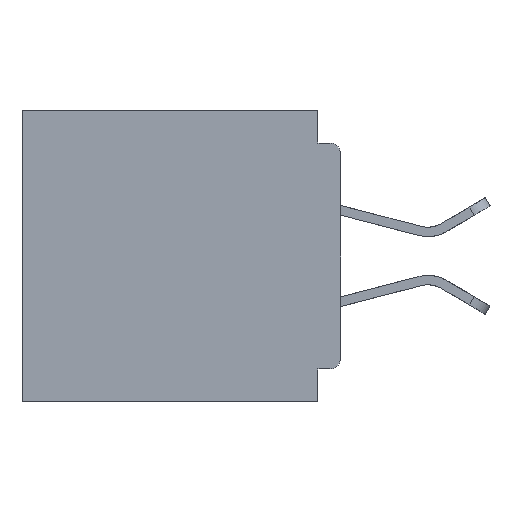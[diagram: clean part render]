
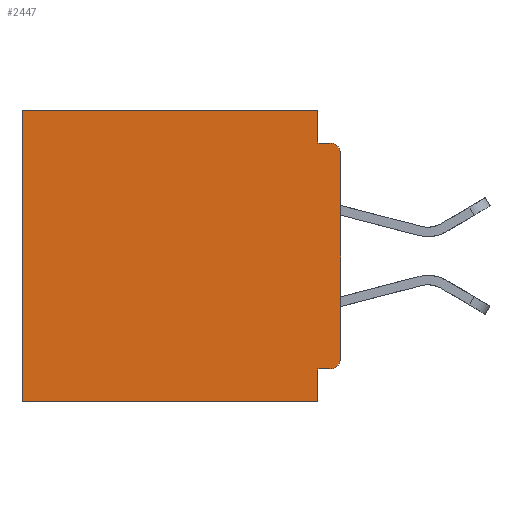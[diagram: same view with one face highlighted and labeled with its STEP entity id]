
A CAD part, left-side view. The second image highlights one B-rep face of the part: STEP entity #2447.
In plain terms, the highlighted planar face has unit normal (-1, 0, 0).
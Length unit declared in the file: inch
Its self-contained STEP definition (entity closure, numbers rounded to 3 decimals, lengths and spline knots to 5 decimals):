
#184 = CARTESIAN_POINT ( 'NONE',  ( 0.3, 0.015, -0.06 ) ) ;
#688 = CARTESIAN_POINT ( 'NONE',  ( 0.3, 0.437, -0.4 ) ) ;
#693 = LINE ( 'NONE', #8231, #17201 ) ;
#1310 = VERTEX_POINT ( 'NONE', #15834 ) ;
#2065 = CARTESIAN_POINT ( 'NONE',  ( 0.3, 0.031, 0. ) ) ;
#2311 = ORIENTED_EDGE ( 'NONE', *, *, #19249, .T. ) ;
#2447 = ADVANCED_FACE ( 'NONE', ( #35693 ), #14220, .F. ) ;
#3426 = CARTESIAN_POINT ( 'NONE',  ( 0.3, 0.437, 0. ) ) ;
#3499 = DIRECTION ( 'NONE',  ( 0., 0., -1. ) ) ;
#3532 = LINE ( 'NONE', #29612, #12281 ) ;
#3850 = ORIENTED_EDGE ( 'NONE', *, *, #18286, .T. ) ;
#3914 = VECTOR ( 'NONE', #31514, 39.37008 ) ;
#6307 = VECTOR ( 'NONE', #27047, 39.37008 ) ;
#6493 = EDGE_CURVE ( 'NONE', #14926, #7414, #3532, .T. ) ;
#6850 = CIRCLE ( 'NONE', #20742, 0.015 ) ;
#7414 = VERTEX_POINT ( 'NONE', #33051 ) ;
#7679 = VERTEX_POINT ( 'NONE', #27681 ) ;
#7861 = ORIENTED_EDGE ( 'NONE', *, *, #28051, .F. ) ;
#8055 = LINE ( 'NONE', #41346, #25611 ) ;
#8152 = VERTEX_POINT ( 'NONE', #17889 ) ;
#8231 = CARTESIAN_POINT ( 'NONE',  ( 0.3, 0., 0. ) ) ;
#8376 = CARTESIAN_POINT ( 'NONE',  ( 0.3, 0.031, 0. ) ) ;
#8762 = CARTESIAN_POINT ( 'NONE',  ( 0.3, 0., -0.4 ) ) ;
#9090 = LINE ( 'NONE', #11339, #25599 ) ;
#9345 = CARTESIAN_POINT ( 'NONE',  ( 0.3, 0., -0.4 ) ) ;
#10101 = DIRECTION ( 'NONE',  ( 1., 0., 0. ) ) ;
#10791 = AXIS2_PLACEMENT_3D ( 'NONE', #184, #23217, #3499 ) ;
#11339 = CARTESIAN_POINT ( 'NONE',  ( 0.3, 0., -0.355 ) ) ;
#11395 = EDGE_CURVE ( 'NONE', #7679, #1310, #9090, .T. ) ;
#11830 = CARTESIAN_POINT ( 'NONE',  ( 0.3, 0., -0.4 ) ) ;
#12067 = DIRECTION ( 'NONE',  ( 0., 0., -1. ) ) ;
#12228 = DIRECTION ( 'NONE',  ( -1., 0., 0. ) ) ;
#12281 = VECTOR ( 'NONE', #29844, 39.37008 ) ;
#12708 = ORIENTED_EDGE ( 'NONE', *, *, #35190, .F. ) ;
#12833 = ORIENTED_EDGE ( 'NONE', *, *, #25616, .F. ) ;
#13420 = VERTEX_POINT ( 'NONE', #3426 ) ;
#14220 = PLANE ( 'NONE',  #16110 ) ;
#14256 = ORIENTED_EDGE ( 'NONE', *, *, #11395, .F. ) ;
#14680 = DIRECTION ( 'NONE',  ( 0., 1., 0. ) ) ;
#14926 = VERTEX_POINT ( 'NONE', #34798 ) ;
#15834 = CARTESIAN_POINT ( 'NONE',  ( 0.3, 0.031, -0.355 ) ) ;
#16017 = DIRECTION ( 'NONE',  ( 0., 0., -1. ) ) ;
#16110 = AXIS2_PLACEMENT_3D ( 'NONE', #8762, #10101, #16213 ) ;
#16213 = DIRECTION ( 'NONE',  ( 0., 0., -1. ) ) ;
#16778 = VERTEX_POINT ( 'NONE', #8376 ) ;
#17102 = EDGE_CURVE ( 'NONE', #36578, #7414, #20330, .T. ) ;
#17201 = VECTOR ( 'NONE', #24676, 39.37008 ) ;
#17889 = CARTESIAN_POINT ( 'NONE',  ( 0.3, 0.031, -0.4 ) ) ;
#18135 = VECTOR ( 'NONE', #16017, 39.37008 ) ;
#18279 = VERTEX_POINT ( 'NONE', #31077 ) ;
#18286 = EDGE_CURVE ( 'NONE', #16778, #13420, #693, .T. ) ;
#18550 = CARTESIAN_POINT ( 'NONE',  ( 0.3, 0.437, -0.4 ) ) ;
#19187 = LINE ( 'NONE', #9345, #18135 ) ;
#19249 = EDGE_CURVE ( 'NONE', #13420, #19551, #41092, .T. ) ;
#19551 = VERTEX_POINT ( 'NONE', #18550 ) ;
#20330 = CIRCLE ( 'NONE', #10791, 0.015 ) ;
#20397 = LINE ( 'NONE', #2065, #3914 ) ;
#20742 = AXIS2_PLACEMENT_3D ( 'NONE', #31883, #12228, #35134 ) ;
#23217 = DIRECTION ( 'NONE',  ( -1., 0., 0. ) ) ;
#23255 = VECTOR ( 'NONE', #31499, 39.37008 ) ;
#24676 = DIRECTION ( 'NONE',  ( 0., 1., 0. ) ) ;
#25599 = VECTOR ( 'NONE', #14680, 39.37008 ) ;
#25611 = VECTOR ( 'NONE', #12067, 39.37008 ) ;
#25616 = EDGE_CURVE ( 'NONE', #36578, #18279, #19187, .T. ) ;
#26516 = CARTESIAN_POINT ( 'NONE',  ( 0.3, 0., -0.06 ) ) ;
#27047 = DIRECTION ( 'NONE',  ( 0., 0., -1. ) ) ;
#27308 = ORIENTED_EDGE ( 'NONE', *, *, #6493, .F. ) ;
#27681 = CARTESIAN_POINT ( 'NONE',  ( 0.3, 0.015, -0.355 ) ) ;
#28051 = EDGE_CURVE ( 'NONE', #16778, #14926, #20397, .T. ) ;
#28535 = EDGE_LOOP ( 'NONE', ( #12833, #32871, #27308, #7861, #3850, #2311, #35212, #12708, #14256, #42350 ) ) ;
#29612 = CARTESIAN_POINT ( 'NONE',  ( 0.3, 0., -0.045 ) ) ;
#29844 = DIRECTION ( 'NONE',  ( 0., -1., 0. ) ) ;
#31077 = CARTESIAN_POINT ( 'NONE',  ( 0.3, 0., -0.34 ) ) ;
#31260 = EDGE_CURVE ( 'NONE', #8152, #19551, #31941, .T. ) ;
#31499 = DIRECTION ( 'NONE',  ( 0., 1., 0. ) ) ;
#31514 = DIRECTION ( 'NONE',  ( 0., 0., -1. ) ) ;
#31883 = CARTESIAN_POINT ( 'NONE',  ( 0.3, 0.015, -0.34 ) ) ;
#31941 = LINE ( 'NONE', #11830, #23255 ) ;
#32871 = ORIENTED_EDGE ( 'NONE', *, *, #17102, .T. ) ;
#33051 = CARTESIAN_POINT ( 'NONE',  ( 0.3, 0.015, -0.045 ) ) ;
#34798 = CARTESIAN_POINT ( 'NONE',  ( 0.3, 0.031, -0.045 ) ) ;
#35134 = DIRECTION ( 'NONE',  ( 0., 0., -1. ) ) ;
#35190 = EDGE_CURVE ( 'NONE', #1310, #8152, #8055, .T. ) ;
#35212 = ORIENTED_EDGE ( 'NONE', *, *, #31260, .F. ) ;
#35693 = FACE_OUTER_BOUND ( 'NONE', #28535, .T. ) ;
#36578 = VERTEX_POINT ( 'NONE', #26516 ) ;
#41028 = EDGE_CURVE ( 'NONE', #7679, #18279, #6850, .T. ) ;
#41092 = LINE ( 'NONE', #688, #6307 ) ;
#41346 = CARTESIAN_POINT ( 'NONE',  ( 0.3, 0.031, -0.4 ) ) ;
#42350 = ORIENTED_EDGE ( 'NONE', *, *, #41028, .T. ) ;
